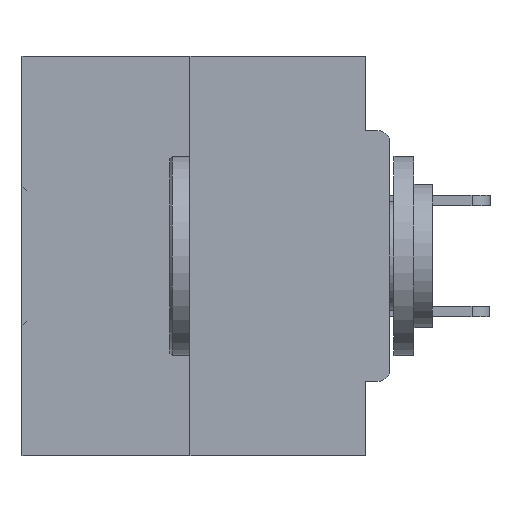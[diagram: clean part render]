
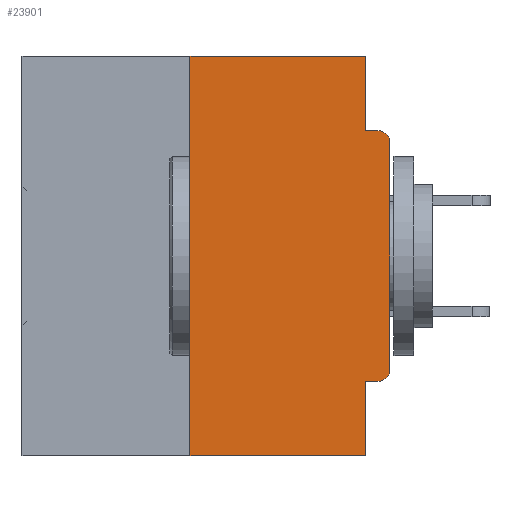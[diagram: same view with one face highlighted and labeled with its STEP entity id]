
A CAD part, left-side view. The second image highlights one B-rep face of the part: STEP entity #23901.
In plain terms, the highlighted planar face has unit normal (-1, 0, 0).
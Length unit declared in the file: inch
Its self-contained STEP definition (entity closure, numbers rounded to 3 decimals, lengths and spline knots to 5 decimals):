
#650 = VERTEX_POINT ( 'NONE', #26419 ) ;
#1124 = DIRECTION ( 'NONE',  ( 0., 0., -1. ) ) ;
#1161 = AXIS2_PLACEMENT_3D ( 'NONE', #16468, #12528, #43581 ) ;
#2089 = CARTESIAN_POINT ( 'NONE',  ( 0., 0.015, -0.4065 ) ) ;
#3052 = EDGE_CURVE ( 'NONE', #40697, #650, #39483, .T. ) ;
#4308 = VERTEX_POINT ( 'NONE', #2089 ) ;
#4961 = ORIENTED_EDGE ( 'NONE', *, *, #25521, .F. ) ;
#5566 = CARTESIAN_POINT ( 'NONE',  ( 0., 0.46, -0.5 ) ) ;
#6937 = EDGE_CURVE ( 'NONE', #23103, #20112, #28500, .T. ) ;
#6940 = CARTESIAN_POINT ( 'NONE',  ( 0., 0., -0.4065 ) ) ;
#6951 = LINE ( 'NONE', #11701, #22021 ) ;
#7003 = ORIENTED_EDGE ( 'NONE', *, *, #23022, .T. ) ;
#7084 = DIRECTION ( 'NONE',  ( 0., 1., 0. ) ) ;
#7231 = CARTESIAN_POINT ( 'NONE',  ( 0., 0.015, -0.1085 ) ) ;
#8023 = VECTOR ( 'NONE', #38657, 39.37008 ) ;
#9001 = DIRECTION ( 'NONE',  ( 0., -1., 0. ) ) ;
#9674 = ORIENTED_EDGE ( 'NONE', *, *, #3052, .T. ) ;
#9843 = CARTESIAN_POINT ( 'NONE',  ( 0., 0., -0.0935 ) ) ;
#9866 = VECTOR ( 'NONE', #9999, 39.37008 ) ;
#9999 = DIRECTION ( 'NONE',  ( 0., -1., 0. ) ) ;
#10477 = ORIENTED_EDGE ( 'NONE', *, *, #25177, .F. ) ;
#10903 = EDGE_LOOP ( 'NONE', ( #24435, #17411, #20064, #10477, #4961, #7003, #39069, #9674, #15723, #16824 ) ) ;
#11190 = CARTESIAN_POINT ( 'NONE',  ( 0., 0.031, -0.5 ) ) ;
#11224 = CIRCLE ( 'NONE', #1161, 0.015 ) ;
#11701 = CARTESIAN_POINT ( 'NONE',  ( 0., 0.25, 0. ) ) ;
#12528 = DIRECTION ( 'NONE',  ( -1., 0., 0. ) ) ;
#13015 = CARTESIAN_POINT ( 'NONE',  ( 0., 0.031, 0. ) ) ;
#13035 = VECTOR ( 'NONE', #35727, 39.37008 ) ;
#13068 = LINE ( 'NONE', #6940, #30279 ) ;
#13572 = VERTEX_POINT ( 'NONE', #32042 ) ;
#14216 = CARTESIAN_POINT ( 'NONE',  ( 0., 0.031, -0.0935 ) ) ;
#14689 = DIRECTION ( 'NONE',  ( 0., 0., -1. ) ) ;
#15723 = ORIENTED_EDGE ( 'NONE', *, *, #24999, .F. ) ;
#16140 = VECTOR ( 'NONE', #9001, 39.37008 ) ;
#16468 = CARTESIAN_POINT ( 'NONE',  ( 0., 0.015, -0.3915 ) ) ;
#16746 = CARTESIAN_POINT ( 'NONE',  ( 0., 0.031, -0.5 ) ) ;
#16824 = ORIENTED_EDGE ( 'NONE', *, *, #37487, .F. ) ;
#16963 = PLANE ( 'NONE',  #34638 ) ;
#17411 = ORIENTED_EDGE ( 'NONE', *, *, #27871, .F. ) ;
#18087 = VECTOR ( 'NONE', #31733, 39.37008 ) ;
#20064 = ORIENTED_EDGE ( 'NONE', *, *, #6937, .T. ) ;
#20112 = VERTEX_POINT ( 'NONE', #16746 ) ;
#21844 = CARTESIAN_POINT ( 'NONE',  ( 0., 0.031, 0. ) ) ;
#22021 = VECTOR ( 'NONE', #42775, 39.37008 ) ;
#22891 = VERTEX_POINT ( 'NONE', #42281 ) ;
#23022 = EDGE_CURVE ( 'NONE', #4308, #37296, #11224, .T. ) ;
#23090 = AXIS2_PLACEMENT_3D ( 'NONE', #7231, #31284, #34748 ) ;
#23103 = VERTEX_POINT ( 'NONE', #40869 ) ;
#23266 = LINE ( 'NONE', #35875, #13035 ) ;
#23901 = ADVANCED_FACE ( 'NONE', ( #39111 ), #16963, .F. ) ;
#24435 = ORIENTED_EDGE ( 'NONE', *, *, #36305, .F. ) ;
#24999 = EDGE_CURVE ( 'NONE', #31776, #650, #43726, .T. ) ;
#25177 = EDGE_CURVE ( 'NONE', #13572, #20112, #40506, .T. ) ;
#25521 = EDGE_CURVE ( 'NONE', #4308, #13572, #13068, .T. ) ;
#25994 = VECTOR ( 'NONE', #14689, 39.37008 ) ;
#26419 = CARTESIAN_POINT ( 'NONE',  ( 0., 0.015, -0.0935 ) ) ;
#27707 = CARTESIAN_POINT ( 'NONE',  ( 0., 0., -0.1085 ) ) ;
#27871 = EDGE_CURVE ( 'NONE', #23103, #22891, #6951, .T. ) ;
#28500 = LINE ( 'NONE', #5566, #16140 ) ;
#29549 = LINE ( 'NONE', #21844, #8023 ) ;
#30279 = VECTOR ( 'NONE', #7084, 39.37008 ) ;
#31284 = DIRECTION ( 'NONE',  ( -1., 0., 0. ) ) ;
#31509 = CARTESIAN_POINT ( 'NONE',  ( 0., 0.46, 0. ) ) ;
#31562 = VERTEX_POINT ( 'NONE', #13015 ) ;
#31733 = DIRECTION ( 'NONE',  ( 0., 0., 1. ) ) ;
#31776 = VERTEX_POINT ( 'NONE', #14216 ) ;
#32042 = CARTESIAN_POINT ( 'NONE',  ( 0., 0.031, -0.4065 ) ) ;
#32047 = CARTESIAN_POINT ( 'NONE',  ( 0., 0., 0. ) ) ;
#34638 = AXIS2_PLACEMENT_3D ( 'NONE', #31509, #38414, #1124 ) ;
#34748 = DIRECTION ( 'NONE',  ( 0., 0., -1. ) ) ;
#35727 = DIRECTION ( 'NONE',  ( 0., -1., 0. ) ) ;
#35875 = CARTESIAN_POINT ( 'NONE',  ( 0., 0.46, 0. ) ) ;
#36305 = EDGE_CURVE ( 'NONE', #22891, #31562, #23266, .T. ) ;
#37296 = VERTEX_POINT ( 'NONE', #39858 ) ;
#37487 = EDGE_CURVE ( 'NONE', #31562, #31776, #29549, .T. ) ;
#38414 = DIRECTION ( 'NONE',  ( 1., 0., 0. ) ) ;
#38471 = LINE ( 'NONE', #32047, #18087 ) ;
#38657 = DIRECTION ( 'NONE',  ( 0., 0., -1. ) ) ;
#39069 = ORIENTED_EDGE ( 'NONE', *, *, #39466, .T. ) ;
#39111 = FACE_OUTER_BOUND ( 'NONE', #10903, .T. ) ;
#39466 = EDGE_CURVE ( 'NONE', #37296, #40697, #38471, .T. ) ;
#39483 = CIRCLE ( 'NONE', #23090, 0.015 ) ;
#39858 = CARTESIAN_POINT ( 'NONE',  ( 0., 0., -0.3915 ) ) ;
#40506 = LINE ( 'NONE', #11190, #25994 ) ;
#40697 = VERTEX_POINT ( 'NONE', #27707 ) ;
#40869 = CARTESIAN_POINT ( 'NONE',  ( 0., 0.25, -0.5 ) ) ;
#42281 = CARTESIAN_POINT ( 'NONE',  ( 0., 0.25, 0. ) ) ;
#42775 = DIRECTION ( 'NONE',  ( 0., 0., 1. ) ) ;
#43581 = DIRECTION ( 'NONE',  ( 0., 0., -1. ) ) ;
#43726 = LINE ( 'NONE', #9843, #9866 ) ;
